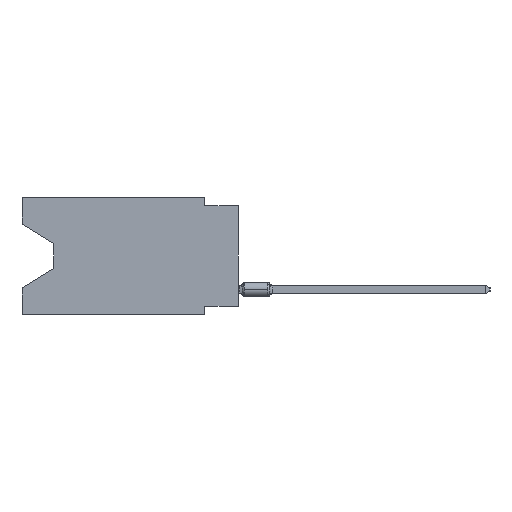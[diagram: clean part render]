
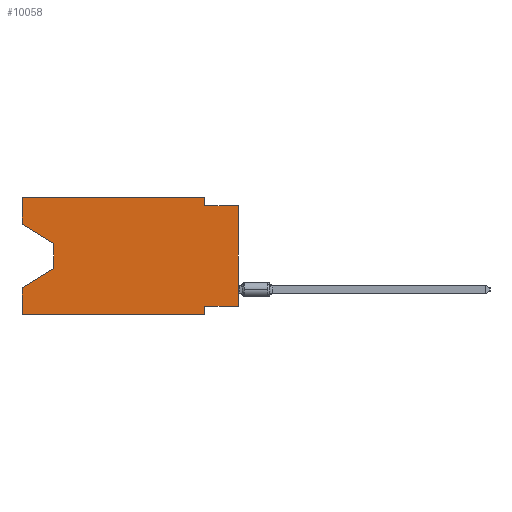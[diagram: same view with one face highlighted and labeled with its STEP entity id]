
A CAD part, left-side view. The second image highlights one B-rep face of the part: STEP entity #10058.
In plain terms, the highlighted planar face has unit normal (-1, 0, 0).
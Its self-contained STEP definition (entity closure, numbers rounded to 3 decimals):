
#220 = DIRECTION ( 'NONE',  ( 0., 0., -1. ) ) ;
#1389 = LINE ( 'NONE', #38463, #25408 ) ;
#1567 = VECTOR ( 'NONE', #30526, 1000. ) ;
#1771 = DIRECTION ( 'NONE',  ( 0., -1., 0. ) ) ;
#3331 = VERTEX_POINT ( 'NONE', #7520 ) ;
#3427 = VECTOR ( 'NONE', #220, 1000. ) ;
#4015 = LINE ( 'NONE', #30506, #39466 ) ;
#4038 = CARTESIAN_POINT ( 'NONE',  ( 0., 0., -0.635 ) ) ;
#4086 = ORIENTED_EDGE ( 'NONE', *, *, #22142, .T. ) ;
#4428 = VECTOR ( 'NONE', #10052, 1000. ) ;
#4573 = CARTESIAN_POINT ( 'NONE',  ( 0., 2.54, 0. ) ) ;
#4724 = LINE ( 'NONE', #18193, #39519 ) ;
#4907 = CARTESIAN_POINT ( 'NONE',  ( 0., 16.383, -2.038 ) ) ;
#5213 = EDGE_CURVE ( 'NONE', #9776, #42020, #18091, .T. ) ;
#6081 = DIRECTION ( 'NONE',  ( 0., 1., 0. ) ) ;
#6542 = EDGE_CURVE ( 'NONE', #32716, #32530, #4724, .T. ) ;
#6940 = ORIENTED_EDGE ( 'NONE', *, *, #12704, .T. ) ;
#7110 = CARTESIAN_POINT ( 'NONE',  ( 0., 16.383, 0. ) ) ;
#7302 = CARTESIAN_POINT ( 'NONE',  ( 0., 13.97, -3.505 ) ) ;
#7391 = EDGE_CURVE ( 'NONE', #32530, #29133, #37162, .T. ) ;
#7464 = CARTESIAN_POINT ( 'NONE',  ( 0., 16.383, 0. ) ) ;
#7520 = CARTESIAN_POINT ( 'NONE',  ( 0., 13.97, -5.385 ) ) ;
#8281 = VERTEX_POINT ( 'NONE', #25142 ) ;
#8519 = EDGE_CURVE ( 'NONE', #14336, #23476, #20765, .T. ) ;
#8762 = DIRECTION ( 'NONE',  ( 0., 0., -1. ) ) ;
#9776 = VERTEX_POINT ( 'NONE', #20057 ) ;
#9812 = CARTESIAN_POINT ( 'NONE',  ( 0., 0., -0.635 ) ) ;
#10052 = DIRECTION ( 'NONE',  ( 0., 0.855, -0.519 ) ) ;
#10058 = ADVANCED_FACE ( 'NONE', ( #25670 ), #21567, .F. ) ;
#10074 = CARTESIAN_POINT ( 'NONE',  ( 0., 16.383, 0. ) ) ;
#10984 = LINE ( 'NONE', #18704, #18745 ) ;
#11086 = ORIENTED_EDGE ( 'NONE', *, *, #6542, .F. ) ;
#11388 = AXIS2_PLACEMENT_3D ( 'NONE', #34798, #18313, #24084 ) ;
#12704 = EDGE_CURVE ( 'NONE', #38033, #3331, #10984, .T. ) ;
#13034 = EDGE_CURVE ( 'NONE', #27482, #15819, #26479, .T. ) ;
#13124 = CARTESIAN_POINT ( 'NONE',  ( 0., 0., 0. ) ) ;
#14024 = DIRECTION ( 'NONE',  ( 0., -0.855, -0.519 ) ) ;
#14336 = VERTEX_POINT ( 'NONE', #15497 ) ;
#14470 = EDGE_CURVE ( 'NONE', #3331, #8281, #40410, .T. ) ;
#15497 = CARTESIAN_POINT ( 'NONE',  ( 0., 2.54, -0.635 ) ) ;
#15819 = VERTEX_POINT ( 'NONE', #37872 ) ;
#16012 = ORIENTED_EDGE ( 'NONE', *, *, #40070, .F. ) ;
#16580 = LINE ( 'NONE', #10074, #24176 ) ;
#16741 = LINE ( 'NONE', #29975, #3427 ) ;
#17456 = DIRECTION ( 'NONE',  ( 0., -1., 0. ) ) ;
#18091 = LINE ( 'NONE', #32155, #18815 ) ;
#18193 = CARTESIAN_POINT ( 'NONE',  ( 0., 16.383, 0. ) ) ;
#18261 = EDGE_CURVE ( 'NONE', #29133, #14336, #1389, .T. ) ;
#18313 = DIRECTION ( 'NONE',  ( 1., 0., 0. ) ) ;
#18704 = CARTESIAN_POINT ( 'NONE',  ( 0., 13.97, -3.505 ) ) ;
#18745 = VECTOR ( 'NONE', #37433, 1000. ) ;
#18815 = VECTOR ( 'NONE', #1771, 1000. ) ;
#20057 = CARTESIAN_POINT ( 'NONE',  ( 0., 16.383, -8.89 ) ) ;
#20765 = LINE ( 'NONE', #4038, #1567 ) ;
#21567 = PLANE ( 'NONE',  #11388 ) ;
#22142 = EDGE_CURVE ( 'NONE', #27482, #23476, #23112, .T. ) ;
#23112 = LINE ( 'NONE', #13124, #33115 ) ;
#23300 = DIRECTION ( 'NONE',  ( 0., 0., 1. ) ) ;
#23438 = ORIENTED_EDGE ( 'NONE', *, *, #5213, .T. ) ;
#23476 = VERTEX_POINT ( 'NONE', #9812 ) ;
#23766 = EDGE_LOOP ( 'NONE', ( #25069, #6940, #40263, #35059, #23438, #16012, #29005, #4086, #24842, #29894, #24877, #11086 ) ) ;
#24084 = DIRECTION ( 'NONE',  ( 0., 0., -1. ) ) ;
#24176 = VECTOR ( 'NONE', #23300, 1000. ) ;
#24842 = ORIENTED_EDGE ( 'NONE', *, *, #8519, .F. ) ;
#24877 = ORIENTED_EDGE ( 'NONE', *, *, #7391, .F. ) ;
#25069 = ORIENTED_EDGE ( 'NONE', *, *, #31762, .T. ) ;
#25142 = CARTESIAN_POINT ( 'NONE',  ( 0., 16.383, -6.852 ) ) ;
#25408 = VECTOR ( 'NONE', #8762, 1000. ) ;
#25670 = FACE_OUTER_BOUND ( 'NONE', #23766, .T. ) ;
#25872 = CARTESIAN_POINT ( 'NONE',  ( 0., 0., -8.255 ) ) ;
#26479 = LINE ( 'NONE', #32545, #31469 ) ;
#27482 = VERTEX_POINT ( 'NONE', #25872 ) ;
#29005 = ORIENTED_EDGE ( 'NONE', *, *, #13034, .F. ) ;
#29133 = VERTEX_POINT ( 'NONE', #4573 ) ;
#29894 = ORIENTED_EDGE ( 'NONE', *, *, #18261, .F. ) ;
#29975 = CARTESIAN_POINT ( 'NONE',  ( 0., 2.54, -8.89 ) ) ;
#30506 = CARTESIAN_POINT ( 'NONE',  ( 0., 16.383, -2.038 ) ) ;
#30526 = DIRECTION ( 'NONE',  ( 0., -1., 0. ) ) ;
#30595 = CARTESIAN_POINT ( 'NONE',  ( 0., 2.54, -8.89 ) ) ;
#31469 = VECTOR ( 'NONE', #6081, 1000. ) ;
#31762 = EDGE_CURVE ( 'NONE', #32716, #38033, #4015, .T. ) ;
#31828 = DIRECTION ( 'NONE',  ( 0., 0., 1. ) ) ;
#32155 = CARTESIAN_POINT ( 'NONE',  ( 0., 16.383, -8.89 ) ) ;
#32530 = VERTEX_POINT ( 'NONE', #7110 ) ;
#32545 = CARTESIAN_POINT ( 'NONE',  ( 0., 0., -8.255 ) ) ;
#32716 = VERTEX_POINT ( 'NONE', #4907 ) ;
#33115 = VECTOR ( 'NONE', #35890, 1000. ) ;
#34798 = CARTESIAN_POINT ( 'NONE',  ( 0., 16.383, 0. ) ) ;
#35059 = ORIENTED_EDGE ( 'NONE', *, *, #42655, .F. ) ;
#35890 = DIRECTION ( 'NONE',  ( 0., 0., 1. ) ) ;
#36294 = CARTESIAN_POINT ( 'NONE',  ( 0., 13.97, -5.385 ) ) ;
#37162 = LINE ( 'NONE', #7464, #42333 ) ;
#37433 = DIRECTION ( 'NONE',  ( 0., 0., -1. ) ) ;
#37872 = CARTESIAN_POINT ( 'NONE',  ( 0., 2.54, -8.255 ) ) ;
#38033 = VERTEX_POINT ( 'NONE', #7302 ) ;
#38463 = CARTESIAN_POINT ( 'NONE',  ( 0., 2.54, 0. ) ) ;
#39466 = VECTOR ( 'NONE', #14024, 1000. ) ;
#39519 = VECTOR ( 'NONE', #31828, 1000. ) ;
#40070 = EDGE_CURVE ( 'NONE', #15819, #42020, #16741, .T. ) ;
#40263 = ORIENTED_EDGE ( 'NONE', *, *, #14470, .T. ) ;
#40410 = LINE ( 'NONE', #36294, #4428 ) ;
#42020 = VERTEX_POINT ( 'NONE', #30595 ) ;
#42333 = VECTOR ( 'NONE', #17456, 1000. ) ;
#42655 = EDGE_CURVE ( 'NONE', #9776, #8281, #16580, .T. ) ;
